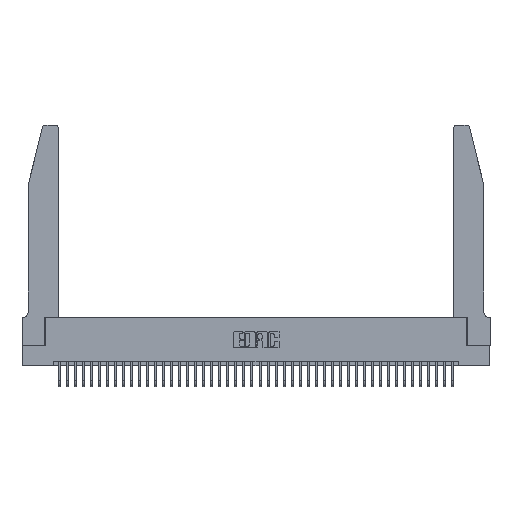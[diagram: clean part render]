
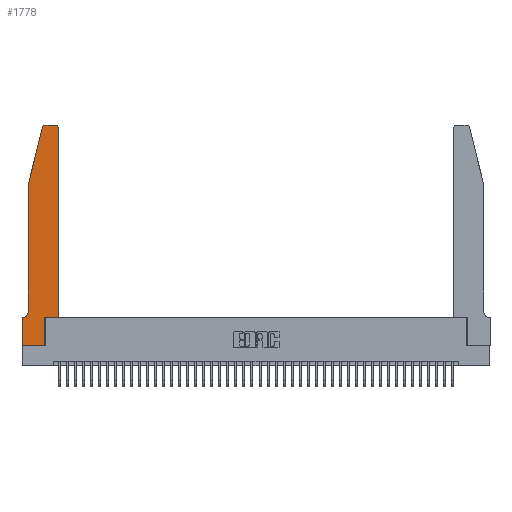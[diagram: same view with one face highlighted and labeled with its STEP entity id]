
A CAD part, top view. The second image highlights one B-rep face of the part: STEP entity #1778.
In plain terms, the highlighted planar face has unit normal (0, 0, 1).
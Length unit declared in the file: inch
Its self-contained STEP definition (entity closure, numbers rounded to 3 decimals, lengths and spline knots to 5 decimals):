
#98 = DIRECTION ( 'NONE',  ( 1., 0., 0. ) ) ;
#524 = CARTESIAN_POINT ( 'NONE',  ( 0.2605, 2.75, 0.37 ) ) ;
#680 = DIRECTION ( 'NONE',  ( -1., 0., 0. ) ) ;
#735 = CARTESIAN_POINT ( 'NONE',  ( 0.284, 2.75, 0.37 ) ) ;
#1778 = ADVANCED_FACE ( 'NONE', ( #29058 ), #10910, .T. ) ;
#1912 = ORIENTED_EDGE ( 'NONE', *, *, #19149, .T. ) ;
#2395 = ORIENTED_EDGE ( 'NONE', *, *, #37669, .T. ) ;
#2492 = CARTESIAN_POINT ( 'NONE',  ( 0.0755, 2., 0.37 ) ) ;
#4125 = DIRECTION ( 'NONE',  ( 1., 0., 0. ) ) ;
#4759 = EDGE_CURVE ( 'NONE', #31373, #5160, #33663, .T. ) ;
#5160 = VERTEX_POINT ( 'NONE', #26107 ) ;
#5756 = CARTESIAN_POINT ( 'NONE',  ( 0.4505, 2.72, 0.37 ) ) ;
#6873 = AXIS2_PLACEMENT_3D ( 'NONE', #11611, #35617, #15077 ) ;
#7087 = CARTESIAN_POINT ( 'NONE',  ( 0.2865, 0.35, 0.37 ) ) ;
#7473 = DIRECTION ( 'NONE',  ( 0., -1., 0. ) ) ;
#8133 = DIRECTION ( 'NONE',  ( 0., 1., 0. ) ) ;
#8374 = ORIENTED_EDGE ( 'NONE', *, *, #31719, .T. ) ;
#8415 = ORIENTED_EDGE ( 'NONE', *, *, #25691, .T. ) ;
#9198 = AXIS2_PLACEMENT_3D ( 'NONE', #34849, #14294, #38280 ) ;
#9772 = VERTEX_POINT ( 'NONE', #39644 ) ;
#10442 = CARTESIAN_POINT ( 'NONE',  ( 0.4505, 0.35, 0.37 ) ) ;
#10597 = ORIENTED_EDGE ( 'NONE', *, *, #20744, .T. ) ;
#10910 = PLANE ( 'NONE',  #43455 ) ;
#11196 = LINE ( 'NONE', #16663, #28352 ) ;
#11611 = CARTESIAN_POINT ( 'NONE',  ( 0.0055, 0.42, 0.37 ) ) ;
#11974 = VECTOR ( 'NONE', #8133, 39.37008 ) ;
#12057 = LINE ( 'NONE', #33194, #20113 ) ;
#12415 = VERTEX_POINT ( 'NONE', #36950 ) ;
#12838 = EDGE_CURVE ( 'NONE', #25911, #42670, #22178, .T. ) ;
#13089 = LINE ( 'NONE', #17621, #39416 ) ;
#13745 = EDGE_LOOP ( 'NONE', ( #35710, #34124, #32543, #8374, #2395, #39534, #8415, #40100, #15974, #1912, #16514, #10597 ) ) ;
#13931 = CIRCLE ( 'NONE', #6873, 0.07 ) ;
#14225 = CARTESIAN_POINT ( 'NONE',  ( 0.4205, 2.72, 0.37 ) ) ;
#14294 = DIRECTION ( 'NONE',  ( 0., 0., 1. ) ) ;
#14789 = VECTOR ( 'NONE', #680, 39.37008 ) ;
#14906 = CARTESIAN_POINT ( 'NONE',  ( 0.4505, 0.35, 0.37 ) ) ;
#15077 = DIRECTION ( 'NONE',  ( -1., 0., 0. ) ) ;
#15263 = LINE ( 'NONE', #524, #14789 ) ;
#15557 = DIRECTION ( 'NONE',  ( 0., -1., 0. ) ) ;
#15658 = CARTESIAN_POINT ( 'NONE',  ( 0.2865, 0., 0.37 ) ) ;
#15974 = ORIENTED_EDGE ( 'NONE', *, *, #4759, .T. ) ;
#16514 = ORIENTED_EDGE ( 'NONE', *, *, #12838, .T. ) ;
#16663 = CARTESIAN_POINT ( 'NONE',  ( 0.0755, 0.35, 0.37 ) ) ;
#17312 = EDGE_CURVE ( 'NONE', #27346, #22997, #13089, .T. ) ;
#17501 = CARTESIAN_POINT ( 'NONE',  ( 0.25487, 2.72718, 0.37 ) ) ;
#17518 = CIRCLE ( 'NONE', #9198, 0.03 ) ;
#17621 = CARTESIAN_POINT ( 'NONE',  ( 0.0755, 2., 0.37 ) ) ;
#17679 = DIRECTION ( 'NONE',  ( 1., 0., 0. ) ) ;
#19149 = EDGE_CURVE ( 'NONE', #5160, #25911, #38765, .T. ) ;
#20113 = VECTOR ( 'NONE', #43504, 39.37008 ) ;
#20744 = EDGE_CURVE ( 'NONE', #42670, #21295, #24971, .T. ) ;
#21259 = CARTESIAN_POINT ( 'NONE',  ( 0., 0.35, 0.37 ) ) ;
#21295 = VERTEX_POINT ( 'NONE', #34885 ) ;
#21338 = VERTEX_POINT ( 'NONE', #35027 ) ;
#22178 = LINE ( 'NONE', #14906, #11974 ) ;
#22997 = VERTEX_POINT ( 'NONE', #2492 ) ;
#24182 = DIRECTION ( 'NONE',  ( 0., 1., 0. ) ) ;
#24502 = LINE ( 'NONE', #39539, #42810 ) ;
#24677 = DIRECTION ( 'NONE',  ( 0., 0., 1. ) ) ;
#24971 = CIRCLE ( 'NONE', #28289, 0.03 ) ;
#24975 = EDGE_CURVE ( 'NONE', #32644, #12415, #11196, .T. ) ;
#25691 = EDGE_CURVE ( 'NONE', #12415, #21338, #24502, .T. ) ;
#25911 = VERTEX_POINT ( 'NONE', #40573 ) ;
#26107 = CARTESIAN_POINT ( 'NONE',  ( 0.2865, 0.35, 0.37 ) ) ;
#26158 = EDGE_CURVE ( 'NONE', #28918, #27346, #17518, .T. ) ;
#26987 = DIRECTION ( 'NONE',  ( -1., 0., 0. ) ) ;
#27346 = VERTEX_POINT ( 'NONE', #17501 ) ;
#27575 = VECTOR ( 'NONE', #7473, 39.37008 ) ;
#28289 = AXIS2_PLACEMENT_3D ( 'NONE', #14225, #38221, #17679 ) ;
#28352 = VECTOR ( 'NONE', #26987, 39.37008 ) ;
#28918 = VERTEX_POINT ( 'NONE', #735 ) ;
#29058 = FACE_OUTER_BOUND ( 'NONE', #13745, .T. ) ;
#29641 = VECTOR ( 'NONE', #98, 39.37008 ) ;
#31129 = EDGE_CURVE ( 'NONE', #21295, #28918, #15263, .T. ) ;
#31280 = DIRECTION ( 'NONE',  ( -0.239, -0.971, 0. ) ) ;
#31373 = VERTEX_POINT ( 'NONE', #15658 ) ;
#31458 = EDGE_CURVE ( 'NONE', #21338, #31373, #12057, .T. ) ;
#31719 = EDGE_CURVE ( 'NONE', #22997, #9772, #36707, .T. ) ;
#32543 = ORIENTED_EDGE ( 'NONE', *, *, #17312, .T. ) ;
#32644 = VERTEX_POINT ( 'NONE', #36220 ) ;
#33194 = CARTESIAN_POINT ( 'NONE',  ( 0., 0., 0.37 ) ) ;
#33663 = LINE ( 'NONE', #7087, #41709 ) ;
#34124 = ORIENTED_EDGE ( 'NONE', *, *, #26158, .T. ) ;
#34849 = CARTESIAN_POINT ( 'NONE',  ( 0.284, 2.72, 0.37 ) ) ;
#34885 = CARTESIAN_POINT ( 'NONE',  ( 0.4205, 2.75, 0.37 ) ) ;
#35027 = CARTESIAN_POINT ( 'NONE',  ( 0., 0., 0.37 ) ) ;
#35617 = DIRECTION ( 'NONE',  ( 0., 0., -1. ) ) ;
#35710 = ORIENTED_EDGE ( 'NONE', *, *, #31129, .T. ) ;
#36220 = CARTESIAN_POINT ( 'NONE',  ( 0.0055, 0.35, 0.37 ) ) ;
#36707 = LINE ( 'NONE', #38085, #27575 ) ;
#36950 = CARTESIAN_POINT ( 'NONE',  ( 0., 0.35, 0.37 ) ) ;
#37669 = EDGE_CURVE ( 'NONE', #9772, #32644, #13931, .T. ) ;
#38085 = CARTESIAN_POINT ( 'NONE',  ( 0.0755, 2., 0.37 ) ) ;
#38221 = DIRECTION ( 'NONE',  ( 0., 0., 1. ) ) ;
#38280 = DIRECTION ( 'NONE',  ( 1., 0., 0. ) ) ;
#38765 = LINE ( 'NONE', #10442, #29641 ) ;
#39416 = VECTOR ( 'NONE', #31280, 39.37008 ) ;
#39534 = ORIENTED_EDGE ( 'NONE', *, *, #24975, .T. ) ;
#39539 = CARTESIAN_POINT ( 'NONE',  ( 0., 0., 0.37 ) ) ;
#39644 = CARTESIAN_POINT ( 'NONE',  ( 0.0755, 0.42, 0.37 ) ) ;
#40100 = ORIENTED_EDGE ( 'NONE', *, *, #31458, .T. ) ;
#40573 = CARTESIAN_POINT ( 'NONE',  ( 0.4505, 0.35, 0.37 ) ) ;
#41709 = VECTOR ( 'NONE', #24182, 39.37008 ) ;
#42670 = VERTEX_POINT ( 'NONE', #5756 ) ;
#42810 = VECTOR ( 'NONE', #15557, 39.37008 ) ;
#43455 = AXIS2_PLACEMENT_3D ( 'NONE', #21259, #24677, #4125 ) ;
#43504 = DIRECTION ( 'NONE',  ( 1., 0., 0. ) ) ;
